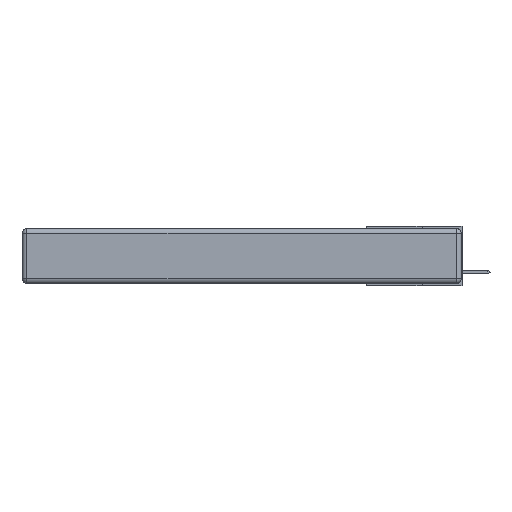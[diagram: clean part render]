
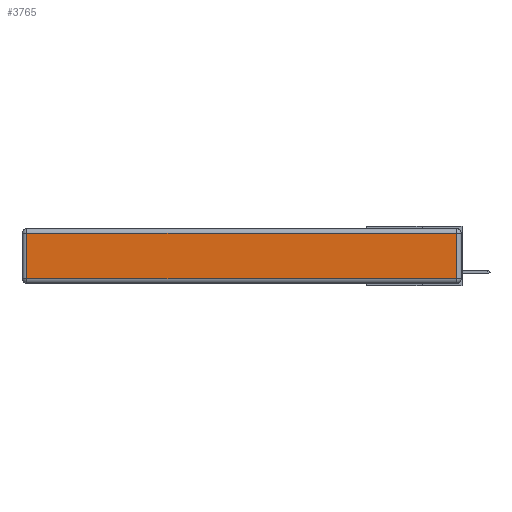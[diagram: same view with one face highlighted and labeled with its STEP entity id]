
A CAD part, left-side view. The second image highlights one B-rep face of the part: STEP entity #3765.
In plain terms, the highlighted planar face has unit normal (-1, 0, 0).
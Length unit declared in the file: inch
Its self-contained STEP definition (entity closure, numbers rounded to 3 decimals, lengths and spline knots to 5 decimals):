
#476 = LINE ( 'NONE', #21408, #10304 ) ;
#816 = ORIENTED_EDGE ( 'NONE', *, *, #19051, .T. ) ;
#2138 = EDGE_LOOP ( 'NONE', ( #8089, #5658, #12594, #816 ) ) ;
#2345 = VERTEX_POINT ( 'NONE', #15455 ) ;
#3384 = EDGE_CURVE ( 'NONE', #8730, #2345, #17051, .T. ) ;
#3765 = ADVANCED_FACE ( 'NONE', ( #15173 ), #19420, .T. ) ;
#5454 = DIRECTION ( 'NONE',  ( 0., 1., 0. ) ) ;
#5658 = ORIENTED_EDGE ( 'NONE', *, *, #21371, .T. ) ;
#5863 = LINE ( 'NONE', #16037, #20036 ) ;
#6160 = DIRECTION ( 'NONE',  ( 0., 0., -1. ) ) ;
#6464 = CARTESIAN_POINT ( 'NONE',  ( 0., 0.03, -0.343 ) ) ;
#8089 = ORIENTED_EDGE ( 'NONE', *, *, #3384, .T. ) ;
#8238 = VERTEX_POINT ( 'NONE', #20063 ) ;
#8730 = VERTEX_POINT ( 'NONE', #19360 ) ;
#9169 = AXIS2_PLACEMENT_3D ( 'NONE', #13714, #11765, #9705 ) ;
#9705 = DIRECTION ( 'NONE',  ( 0., 0., 1. ) ) ;
#10304 = VECTOR ( 'NONE', #5454, 39.37008 ) ;
#10986 = CARTESIAN_POINT ( 'NONE',  ( 0., 0.03, -0.03 ) ) ;
#11765 = DIRECTION ( 'NONE',  ( -1., 0., 0. ) ) ;
#12594 = ORIENTED_EDGE ( 'NONE', *, *, #14953, .T. ) ;
#13177 = LINE ( 'NONE', #6464, #22462 ) ;
#13714 = CARTESIAN_POINT ( 'NONE',  ( 0., 0., -0.343 ) ) ;
#14432 = CARTESIAN_POINT ( 'NONE',  ( 0., 0., -0.313 ) ) ;
#14953 = EDGE_CURVE ( 'NONE', #19135, #8238, #476, .T. ) ;
#15173 = FACE_OUTER_BOUND ( 'NONE', #2138, .T. ) ;
#15455 = CARTESIAN_POINT ( 'NONE',  ( 0., 0.03, -0.313 ) ) ;
#16037 = CARTESIAN_POINT ( 'NONE',  ( 0., 2.72, -0.343 ) ) ;
#17051 = LINE ( 'NONE', #14432, #19203 ) ;
#19051 = EDGE_CURVE ( 'NONE', #8238, #8730, #5863, .T. ) ;
#19135 = VERTEX_POINT ( 'NONE', #10986 ) ;
#19203 = VECTOR ( 'NONE', #24376, 39.37008 ) ;
#19360 = CARTESIAN_POINT ( 'NONE',  ( 0., 2.72, -0.313 ) ) ;
#19420 = PLANE ( 'NONE',  #9169 ) ;
#20036 = VECTOR ( 'NONE', #6160, 39.37008 ) ;
#20063 = CARTESIAN_POINT ( 'NONE',  ( 0., 2.72, -0.03 ) ) ;
#21371 = EDGE_CURVE ( 'NONE', #2345, #19135, #13177, .T. ) ;
#21408 = CARTESIAN_POINT ( 'NONE',  ( 0., 2.75, -0.03 ) ) ;
#22323 = DIRECTION ( 'NONE',  ( 0., 0., 1. ) ) ;
#22462 = VECTOR ( 'NONE', #22323, 39.37008 ) ;
#24376 = DIRECTION ( 'NONE',  ( 0., -1., 0. ) ) ;
